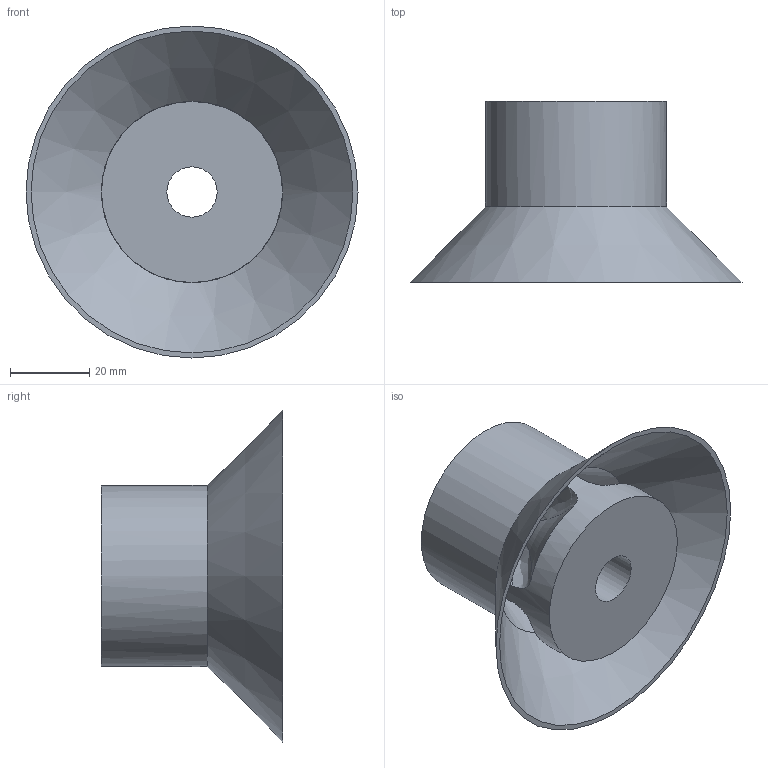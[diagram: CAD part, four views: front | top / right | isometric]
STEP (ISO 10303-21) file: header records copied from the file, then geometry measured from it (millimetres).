
FILE_DESCRIPTION(/* description */ (''),/* implementation_level */ '2;1');
FILE_NAME(/* name */ '1.8 Dia 50 CAL Baffle STEP.step',/* time_stamp */ '2019-06-01T15:56:55-04:00',/* author */ (''),/* organization */ (''),/* preprocessor_version */ 'ST-DEVELOPER v18',/* originating_system */ 'Autodesk Translation Framework v8.2.0.1029',/* authorisation */ '');
FILE_SCHEMA (('AUTOMOTIVE_DESIGN { 1 0 10303 214 3 1 1 }'));
Length unit declared in the file: inch
Products named in the file (1): baf 7 50 cal
Bounding box: 83.82 x 45.72 x 83.82 mm (x, y, z)
Volume: 56534.7 mm3; surface area: 26117.5 mm2
Topology: 1 solids, 1 shells, 36 faces, 126 edges, 85 vertices
Faces by surface type: plane 15, bspline 13, cylinder 4, cone 2, torus 2
Full cylindrical faces by diameter (mm): 12.7 x2, 45.72 x2
Entity records: 2387 total; most frequent: CARTESIAN_POINT 1396, ORIENTED_EDGE 252, DIRECTION 136, EDGE_CURVE 126, VERTEX_POINT 85, B_SPLINE_CURVE_WITH_KNOTS 70, AXIS2_PLACEMENT_3D 57, EDGE_LOOP 39
